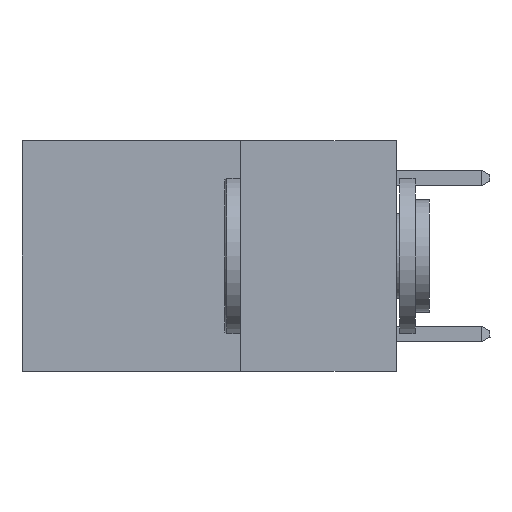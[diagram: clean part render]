
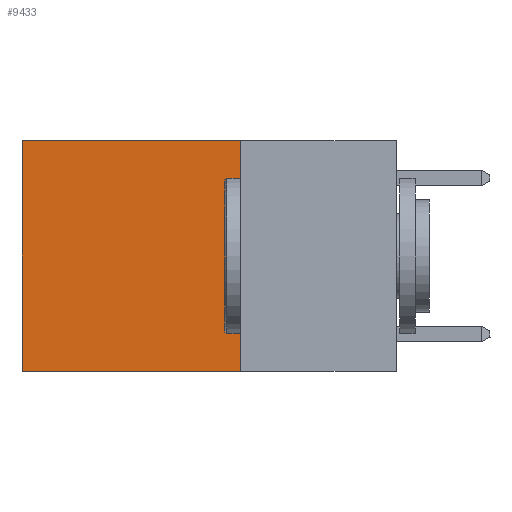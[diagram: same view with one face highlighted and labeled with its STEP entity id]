
A CAD part, left-side view. The second image highlights one B-rep face of the part: STEP entity #9433.
In plain terms, the highlighted planar face has unit normal (-1, 0, 0).
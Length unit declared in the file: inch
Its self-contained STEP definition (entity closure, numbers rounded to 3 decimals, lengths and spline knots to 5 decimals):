
#727 = DIRECTION ( 'NONE',  ( 0., 1., 0. ) ) ;
#953 = AXIS2_PLACEMENT_3D ( 'NONE', #2029, #16986, #6132 ) ;
#1022 = CARTESIAN_POINT ( 'NONE',  ( 0.2625, 0.6, 0. ) ) ;
#1073 = CARTESIAN_POINT ( 'NONE',  ( 0.2625, 0.6, -0.37 ) ) ;
#1203 = VECTOR ( 'NONE', #4096, 39.37008 ) ;
#1233 = LINE ( 'NONE', #18527, #1203 ) ;
#1299 = EDGE_CURVE ( 'NONE', #15271, #13605, #19534, .T. ) ;
#1644 = EDGE_CURVE ( 'NONE', #4541, #13605, #17535, .T. ) ;
#1947 = EDGE_LOOP ( 'NONE', ( #6919, #7486, #7794, #8000 ) ) ;
#1996 = VERTEX_POINT ( 'NONE', #8896 ) ;
#2029 = CARTESIAN_POINT ( 'NONE',  ( 0.2625, 0.25, 0. ) ) ;
#4096 = DIRECTION ( 'NONE',  ( 0., 0., -1. ) ) ;
#4221 = PLANE ( 'NONE',  #953 ) ;
#4541 = VERTEX_POINT ( 'NONE', #6524 ) ;
#4604 = EDGE_CURVE ( 'NONE', #1996, #15271, #13545, .T. ) ;
#6132 = DIRECTION ( 'NONE',  ( 0., 0., -1. ) ) ;
#6524 = CARTESIAN_POINT ( 'NONE',  ( 0.2625, 0.25, -0.37 ) ) ;
#6919 = ORIENTED_EDGE ( 'NONE', *, *, #1299, .T. ) ;
#7486 = ORIENTED_EDGE ( 'NONE', *, *, #1644, .F. ) ;
#7794 = ORIENTED_EDGE ( 'NONE', *, *, #15692, .F. ) ;
#8000 = ORIENTED_EDGE ( 'NONE', *, *, #4604, .T. ) ;
#8896 = CARTESIAN_POINT ( 'NONE',  ( 0.2625, 0.25, 0. ) ) ;
#9433 = ADVANCED_FACE ( 'NONE', ( #19320 ), #4221, .F. ) ;
#13545 = LINE ( 'NONE', #20885, #13606 ) ;
#13605 = VERTEX_POINT ( 'NONE', #1073 ) ;
#13606 = VECTOR ( 'NONE', #727, 39.37008 ) ;
#15271 = VERTEX_POINT ( 'NONE', #1022 ) ;
#15404 = DIRECTION ( 'NONE',  ( 0., 1., 0. ) ) ;
#15410 = CARTESIAN_POINT ( 'NONE',  ( 0.2625, 0.25, -0.37 ) ) ;
#15692 = EDGE_CURVE ( 'NONE', #1996, #4541, #1233, .T. ) ;
#16986 = DIRECTION ( 'NONE',  ( 1., 0., 0. ) ) ;
#17535 = LINE ( 'NONE', #15410, #17669 ) ;
#17669 = VECTOR ( 'NONE', #15404, 39.37008 ) ;
#18527 = CARTESIAN_POINT ( 'NONE',  ( 0.2625, 0.25, 0. ) ) ;
#19320 = FACE_OUTER_BOUND ( 'NONE', #1947, .T. ) ;
#19477 = VECTOR ( 'NONE', #21127, 39.37008 ) ;
#19534 = LINE ( 'NONE', #21097, #19477 ) ;
#20885 = CARTESIAN_POINT ( 'NONE',  ( 0.2625, 0.25, 0. ) ) ;
#21097 = CARTESIAN_POINT ( 'NONE',  ( 0.2625, 0.6, 0. ) ) ;
#21127 = DIRECTION ( 'NONE',  ( 0., 0., -1. ) ) ;
